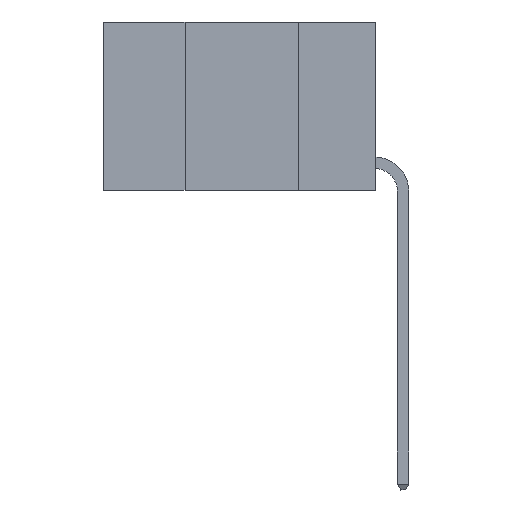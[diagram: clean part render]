
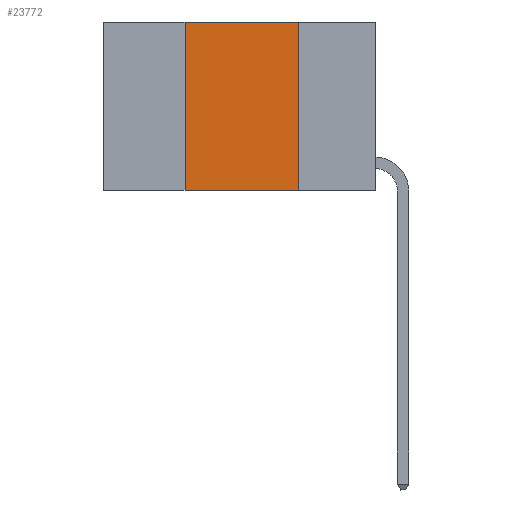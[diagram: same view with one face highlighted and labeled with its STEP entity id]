
A CAD part, left-side view. The second image highlights one B-rep face of the part: STEP entity #23772.
In plain terms, the highlighted planar face has unit normal (-1, 0, 0).
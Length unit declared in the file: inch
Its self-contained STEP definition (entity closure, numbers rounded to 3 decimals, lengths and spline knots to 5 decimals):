
#784 = CARTESIAN_POINT ( 'NONE',  ( 0., 0.17, 0. ) ) ;
#1425 = CARTESIAN_POINT ( 'NONE',  ( 0., 0.6, 0. ) ) ;
#1510 = EDGE_CURVE ( 'NONE', #15136, #19286, #11251, .T. ) ;
#2600 = CARTESIAN_POINT ( 'NONE',  ( 0., 0.42, 0. ) ) ;
#3719 = FACE_OUTER_BOUND ( 'NONE', #5739, .T. ) ;
#4914 = LINE ( 'NONE', #9634, #16517 ) ;
#5739 = EDGE_LOOP ( 'NONE', ( #20351, #8433, #13055, #29586 ) ) ;
#7278 = EDGE_CURVE ( 'NONE', #25406, #19286, #4914, .T. ) ;
#7580 = VECTOR ( 'NONE', #17961, 39.37008 ) ;
#8433 = ORIENTED_EDGE ( 'NONE', *, *, #18659, .F. ) ;
#8650 = CARTESIAN_POINT ( 'NONE',  ( 0., 0.17, 0. ) ) ;
#9634 = CARTESIAN_POINT ( 'NONE',  ( 0., 0.6, -0.37 ) ) ;
#9652 = EDGE_CURVE ( 'NONE', #25406, #30046, #16925, .T. ) ;
#10451 = CARTESIAN_POINT ( 'NONE',  ( 0., 0.17, -0.37 ) ) ;
#11251 = LINE ( 'NONE', #8650, #7580 ) ;
#12186 = CARTESIAN_POINT ( 'NONE',  ( 0., 0.42, 0. ) ) ;
#13055 = ORIENTED_EDGE ( 'NONE', *, *, #9652, .F. ) ;
#15136 = VERTEX_POINT ( 'NONE', #784 ) ;
#16517 = VECTOR ( 'NONE', #16965, 39.37008 ) ;
#16925 = LINE ( 'NONE', #12186, #27672 ) ;
#16965 = DIRECTION ( 'NONE',  ( 0., -1., 0. ) ) ;
#17075 = DIRECTION ( 'NONE',  ( 0., -1., 0. ) ) ;
#17377 = CARTESIAN_POINT ( 'NONE',  ( 0., 0.6, 0. ) ) ;
#17961 = DIRECTION ( 'NONE',  ( 0., 0., -1. ) ) ;
#18659 = EDGE_CURVE ( 'NONE', #30046, #15136, #23913, .T. ) ;
#19286 = VERTEX_POINT ( 'NONE', #10451 ) ;
#19365 = CARTESIAN_POINT ( 'NONE',  ( 0., 0.42, -0.37 ) ) ;
#20351 = ORIENTED_EDGE ( 'NONE', *, *, #1510, .F. ) ;
#21767 = DIRECTION ( 'NONE',  ( 0., 0., 1. ) ) ;
#22301 = PLANE ( 'NONE',  #27051 ) ;
#22540 = VECTOR ( 'NONE', #17075, 39.37008 ) ;
#23772 = ADVANCED_FACE ( 'NONE', ( #3719 ), #22301, .F. ) ;
#23913 = LINE ( 'NONE', #17377, #22540 ) ;
#24752 = DIRECTION ( 'NONE',  ( 0., 0., -1. ) ) ;
#25406 = VERTEX_POINT ( 'NONE', #19365 ) ;
#27051 = AXIS2_PLACEMENT_3D ( 'NONE', #1425, #29311, #24752 ) ;
#27672 = VECTOR ( 'NONE', #21767, 39.37008 ) ;
#29311 = DIRECTION ( 'NONE',  ( 1., 0., 0. ) ) ;
#29586 = ORIENTED_EDGE ( 'NONE', *, *, #7278, .T. ) ;
#30046 = VERTEX_POINT ( 'NONE', #2600 ) ;
